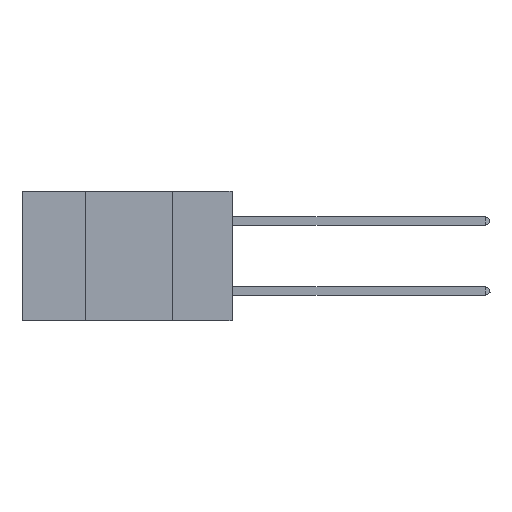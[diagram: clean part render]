
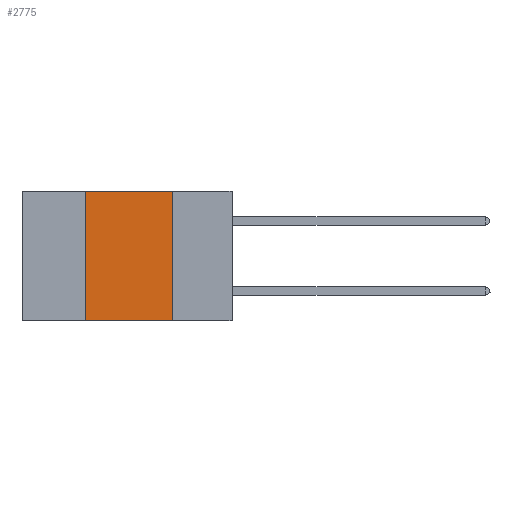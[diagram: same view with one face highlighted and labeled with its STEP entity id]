
A CAD part, left-side view. The second image highlights one B-rep face of the part: STEP entity #2775.
In plain terms, the highlighted planar face has unit normal (-1, 0, 0).
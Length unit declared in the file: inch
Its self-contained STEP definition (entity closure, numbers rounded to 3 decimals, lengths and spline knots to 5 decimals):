
#61 = EDGE_CURVE ( 'NONE', #13963, #2954, #3589, .T. ) ;
#1119 = CARTESIAN_POINT ( 'NONE',  ( 0., 0.6, -0.37 ) ) ;
#1166 = AXIS2_PLACEMENT_3D ( 'NONE', #8316, #6597, #5515 ) ;
#1607 = DIRECTION ( 'NONE',  ( 0., -1., 0. ) ) ;
#1886 = CARTESIAN_POINT ( 'NONE',  ( 0., 0.17, 0. ) ) ;
#2519 = LINE ( 'NONE', #1886, #15423 ) ;
#2604 = DIRECTION ( 'NONE',  ( 0., -1., 0. ) ) ;
#2775 = ADVANCED_FACE ( 'NONE', ( #9989 ), #14635, .F. ) ;
#2954 = VERTEX_POINT ( 'NONE', #4756 ) ;
#3255 = ORIENTED_EDGE ( 'NONE', *, *, #5555, .F. ) ;
#3347 = EDGE_CURVE ( 'NONE', #5878, #13378, #11915, .T. ) ;
#3498 = VECTOR ( 'NONE', #1607, 39.37008 ) ;
#3589 = LINE ( 'NONE', #1119, #6761 ) ;
#4123 = EDGE_LOOP ( 'NONE', ( #6432, #13267, #3255, #14580 ) ) ;
#4501 = CARTESIAN_POINT ( 'NONE',  ( 0., 0.42, 0. ) ) ;
#4756 = CARTESIAN_POINT ( 'NONE',  ( 0., 0.17, -0.37 ) ) ;
#5515 = DIRECTION ( 'NONE',  ( 0., 0., -1. ) ) ;
#5555 = EDGE_CURVE ( 'NONE', #13963, #5878, #14165, .T. ) ;
#5639 = DIRECTION ( 'NONE',  ( 0., 0., -1. ) ) ;
#5788 = CARTESIAN_POINT ( 'NONE',  ( 0., 0.17, 0. ) ) ;
#5878 = VERTEX_POINT ( 'NONE', #4501 ) ;
#6196 = VECTOR ( 'NONE', #14054, 39.37008 ) ;
#6432 = ORIENTED_EDGE ( 'NONE', *, *, #14830, .F. ) ;
#6556 = CARTESIAN_POINT ( 'NONE',  ( 0., 0.42, -0.37 ) ) ;
#6597 = DIRECTION ( 'NONE',  ( 1., 0., 0. ) ) ;
#6761 = VECTOR ( 'NONE', #2604, 39.37008 ) ;
#8316 = CARTESIAN_POINT ( 'NONE',  ( 0., 0.6, 0. ) ) ;
#9989 = FACE_OUTER_BOUND ( 'NONE', #4123, .T. ) ;
#11915 = LINE ( 'NONE', #15138, #3498 ) ;
#13267 = ORIENTED_EDGE ( 'NONE', *, *, #3347, .F. ) ;
#13378 = VERTEX_POINT ( 'NONE', #5788 ) ;
#13963 = VERTEX_POINT ( 'NONE', #6556 ) ;
#14054 = DIRECTION ( 'NONE',  ( 0., 0., 1. ) ) ;
#14165 = LINE ( 'NONE', #15078, #6196 ) ;
#14580 = ORIENTED_EDGE ( 'NONE', *, *, #61, .T. ) ;
#14635 = PLANE ( 'NONE',  #1166 ) ;
#14830 = EDGE_CURVE ( 'NONE', #13378, #2954, #2519, .T. ) ;
#15078 = CARTESIAN_POINT ( 'NONE',  ( 0., 0.42, 0. ) ) ;
#15138 = CARTESIAN_POINT ( 'NONE',  ( 0., 0.6, 0. ) ) ;
#15423 = VECTOR ( 'NONE', #5639, 39.37008 ) ;
